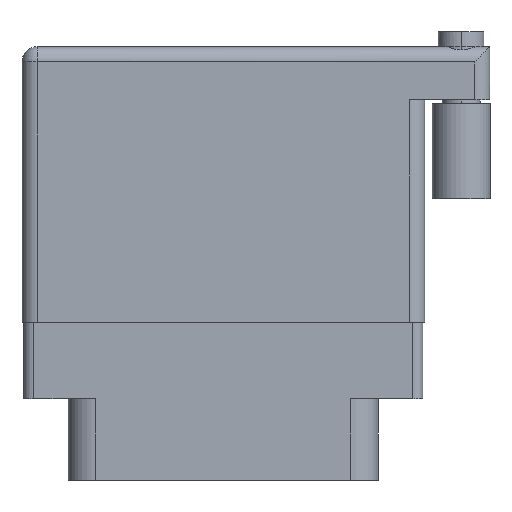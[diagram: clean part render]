
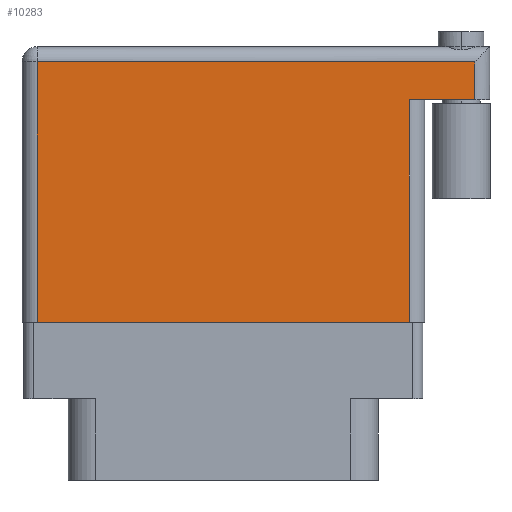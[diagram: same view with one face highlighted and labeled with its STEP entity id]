
A CAD part, front view. The second image highlights one B-rep face of the part: STEP entity #10283.
In plain terms, the highlighted face is planar.
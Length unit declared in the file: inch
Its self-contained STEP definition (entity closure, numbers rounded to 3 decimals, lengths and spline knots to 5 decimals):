
#28 = CARTESIAN_POINT ( 'NONE',  ( 0., 0.906, 0. ) ) ;
#355 = EDGE_LOOP ( 'NONE', ( #11376, #11333, #16648, #4780, #1781, #939 ) ) ;
#612 = CARTESIAN_POINT ( 'NONE',  ( 1.489, 0.856, 0. ) ) ;
#939 = ORIENTED_EDGE ( 'NONE', *, *, #18400, .T. ) ;
#1781 = ORIENTED_EDGE ( 'NONE', *, *, #6542, .T. ) ;
#1868 = DIRECTION ( 'NONE',  ( 0., 1., 0. ) ) ;
#2441 = EDGE_CURVE ( 'NONE', #17311, #3919, #15170, .T. ) ;
#2841 = VECTOR ( 'NONE', #5870, 39.37008 ) ;
#3195 = DIRECTION ( 'NONE',  ( -1., 0., 0. ) ) ;
#3750 = CARTESIAN_POINT ( 'NONE',  ( 0., 0., 0. ) ) ;
#3879 = EDGE_CURVE ( 'NONE', #16719, #3919, #18854, .T. ) ;
#3919 = VERTEX_POINT ( 'NONE', #21527 ) ;
#4780 = ORIENTED_EDGE ( 'NONE', *, *, #16510, .T. ) ;
#5216 = VECTOR ( 'NONE', #9796, 39.37008 ) ;
#5790 = VERTEX_POINT ( 'NONE', #6262 ) ;
#5870 = DIRECTION ( 'NONE',  ( 0., -1., 0. ) ) ;
#6215 = CARTESIAN_POINT ( 'NONE',  ( 1.275, 0.731, 0. ) ) ;
#6262 = CARTESIAN_POINT ( 'NONE',  ( 0.05, 0., 0. ) ) ;
#6542 = EDGE_CURVE ( 'NONE', #10124, #10039, #17699, .T. ) ;
#6562 = CARTESIAN_POINT ( 'NONE',  ( 1.539, 0.731, 0. ) ) ;
#8685 = DIRECTION ( 'NONE',  ( 0., 0., -1. ) ) ;
#8825 = CARTESIAN_POINT ( 'NONE',  ( 0.05, 0.856, 0. ) ) ;
#9127 = VECTOR ( 'NONE', #18213, 39.37008 ) ;
#9508 = VECTOR ( 'NONE', #3195, 39.37008 ) ;
#9796 = DIRECTION ( 'NONE',  ( 0., 1., 0. ) ) ;
#9989 = EDGE_CURVE ( 'NONE', #5790, #16719, #17284, .T. ) ;
#10039 = VERTEX_POINT ( 'NONE', #8825 ) ;
#10124 = VERTEX_POINT ( 'NONE', #612 ) ;
#10283 = ADVANCED_FACE ( 'NONE', ( #16494 ), #15367, .F. ) ;
#11333 = ORIENTED_EDGE ( 'NONE', *, *, #3879, .T. ) ;
#11376 = ORIENTED_EDGE ( 'NONE', *, *, #9989, .T. ) ;
#13042 = VECTOR ( 'NONE', #20805, 39.37008 ) ;
#13137 = CARTESIAN_POINT ( 'NONE',  ( 0., 0.856, 0. ) ) ;
#13782 = LINE ( 'NONE', #19328, #2841 ) ;
#13910 = DIRECTION ( 'NONE',  ( -1., 0., 0. ) ) ;
#14324 = CARTESIAN_POINT ( 'NONE',  ( 1.275, 0., 0. ) ) ;
#14954 = VECTOR ( 'NONE', #1868, 39.37008 ) ;
#15170 = LINE ( 'NONE', #6562, #9508 ) ;
#15367 = PLANE ( 'NONE',  #19689 ) ;
#16494 = FACE_OUTER_BOUND ( 'NONE', #355, .T. ) ;
#16510 = EDGE_CURVE ( 'NONE', #17311, #10124, #17072, .T. ) ;
#16648 = ORIENTED_EDGE ( 'NONE', *, *, #2441, .F. ) ;
#16719 = VERTEX_POINT ( 'NONE', #14324 ) ;
#17072 = LINE ( 'NONE', #18985, #14954 ) ;
#17284 = LINE ( 'NONE', #3750, #13042 ) ;
#17311 = VERTEX_POINT ( 'NONE', #18982 ) ;
#17699 = LINE ( 'NONE', #13137, #9127 ) ;
#18213 = DIRECTION ( 'NONE',  ( -1., 0., 0. ) ) ;
#18400 = EDGE_CURVE ( 'NONE', #10039, #5790, #13782, .T. ) ;
#18854 = LINE ( 'NONE', #6215, #5216 ) ;
#18982 = CARTESIAN_POINT ( 'NONE',  ( 1.489, 0.731, 0. ) ) ;
#18985 = CARTESIAN_POINT ( 'NONE',  ( 1.489, 0.906, 0. ) ) ;
#19328 = CARTESIAN_POINT ( 'NONE',  ( 0.05, 0., 0. ) ) ;
#19689 = AXIS2_PLACEMENT_3D ( 'NONE', #28, #8685, #13910 ) ;
#20805 = DIRECTION ( 'NONE',  ( 1., 0., 0. ) ) ;
#21527 = CARTESIAN_POINT ( 'NONE',  ( 1.275, 0.731, 0. ) ) ;
